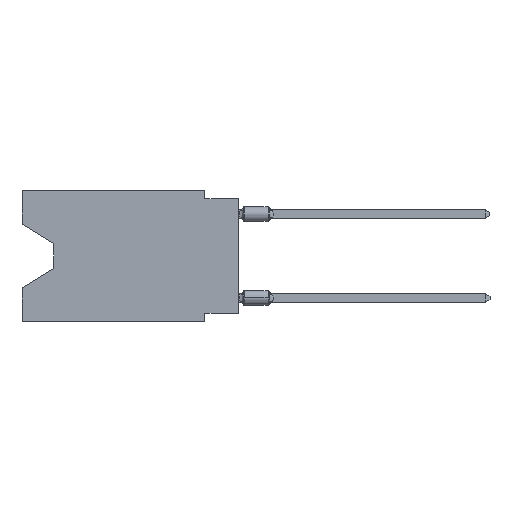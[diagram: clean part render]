
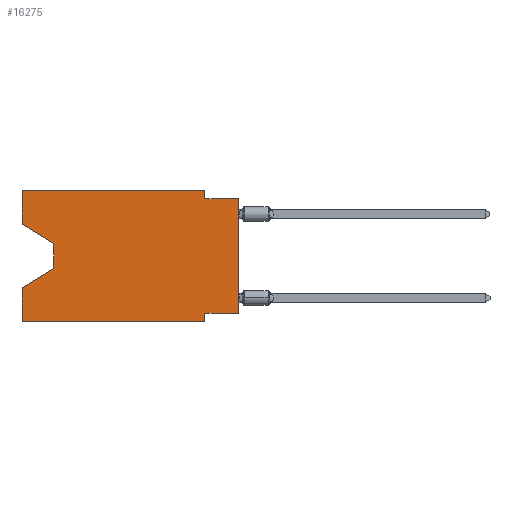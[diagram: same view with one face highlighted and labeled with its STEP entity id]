
A CAD part, left-side view. The second image highlights one B-rep face of the part: STEP entity #16275.
In plain terms, the highlighted planar face has unit normal (-1, 0, 0).
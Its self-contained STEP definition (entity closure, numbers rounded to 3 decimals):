
#249 = PLANE ( 'NONE',  #9242 ) ;
#339 = DIRECTION ( 'NONE',  ( 0., 0., 1. ) ) ;
#496 = CARTESIAN_POINT ( 'NONE',  ( 0., 2.54, -9.906 ) ) ;
#578 = LINE ( 'NONE', #17712, #9018 ) ;
#1679 = CARTESIAN_POINT ( 'NONE',  ( 0., 16.383, 0. ) ) ;
#2886 = EDGE_CURVE ( 'NONE', #3172, #21950, #13737, .T. ) ;
#3172 = VERTEX_POINT ( 'NONE', #18987 ) ;
#3490 = ORIENTED_EDGE ( 'NONE', *, *, #15103, .T. ) ;
#3615 = LINE ( 'NONE', #1679, #9831 ) ;
#3738 = CARTESIAN_POINT ( 'NONE',  ( 0., 0., 0. ) ) ;
#3772 = CARTESIAN_POINT ( 'NONE',  ( 0., 13.97, -4.013 ) ) ;
#3901 = CARTESIAN_POINT ( 'NONE',  ( 0., 16.383, 0. ) ) ;
#4008 = ORIENTED_EDGE ( 'NONE', *, *, #5874, .F. ) ;
#4111 = VECTOR ( 'NONE', #16058, 1000. ) ;
#4529 = CARTESIAN_POINT ( 'NONE',  ( 0., 0., -9.271 ) ) ;
#4678 = DIRECTION ( 'NONE',  ( 0., 0., -1. ) ) ;
#5104 = VECTOR ( 'NONE', #5360, 1000. ) ;
#5166 = CARTESIAN_POINT ( 'NONE',  ( 0., 16.383, 0. ) ) ;
#5337 = VECTOR ( 'NONE', #9088, 1000. ) ;
#5360 = DIRECTION ( 'NONE',  ( 0., -0.855, -0.519 ) ) ;
#5420 = EDGE_CURVE ( 'NONE', #3172, #15425, #14476, .T. ) ;
#5471 = DIRECTION ( 'NONE',  ( 0., 0., -1. ) ) ;
#5735 = DIRECTION ( 'NONE',  ( 1., 0., 0. ) ) ;
#5796 = CARTESIAN_POINT ( 'NONE',  ( 0., 2.54, 0. ) ) ;
#5874 = EDGE_CURVE ( 'NONE', #21510, #11954, #22723, .T. ) ;
#6277 = CARTESIAN_POINT ( 'NONE',  ( 0., 13.97, -4.013 ) ) ;
#6551 = EDGE_CURVE ( 'NONE', #12449, #8440, #20312, .T. ) ;
#7234 = ORIENTED_EDGE ( 'NONE', *, *, #23319, .F. ) ;
#7327 = LINE ( 'NONE', #12842, #19570 ) ;
#7402 = DIRECTION ( 'NONE',  ( 0., 1., 0. ) ) ;
#7459 = VERTEX_POINT ( 'NONE', #9820 ) ;
#7668 = DIRECTION ( 'NONE',  ( 0., 0., 1. ) ) ;
#7743 = ORIENTED_EDGE ( 'NONE', *, *, #16140, .T. ) ;
#7904 = ORIENTED_EDGE ( 'NONE', *, *, #10809, .T. ) ;
#7913 = LINE ( 'NONE', #3738, #8195 ) ;
#8195 = VECTOR ( 'NONE', #7668, 1000. ) ;
#8241 = LINE ( 'NONE', #6277, #9632 ) ;
#8387 = DIRECTION ( 'NONE',  ( 0., 0., -1. ) ) ;
#8440 = VERTEX_POINT ( 'NONE', #18063 ) ;
#8969 = FACE_OUTER_BOUND ( 'NONE', #14209, .T. ) ;
#9018 = VECTOR ( 'NONE', #8387, 1000. ) ;
#9088 = DIRECTION ( 'NONE',  ( 0., 0., 1. ) ) ;
#9242 = AXIS2_PLACEMENT_3D ( 'NONE', #3901, #5735, #16195 ) ;
#9350 = CARTESIAN_POINT ( 'NONE',  ( 0., 16.383, 0. ) ) ;
#9607 = EDGE_CURVE ( 'NONE', #21632, #20937, #3615, .T. ) ;
#9632 = VECTOR ( 'NONE', #4678, 1000. ) ;
#9792 = ORIENTED_EDGE ( 'NONE', *, *, #2886, .T. ) ;
#9820 = CARTESIAN_POINT ( 'NONE',  ( 0., 13.97, -5.893 ) ) ;
#9831 = VECTOR ( 'NONE', #339, 1000. ) ;
#10738 = CARTESIAN_POINT ( 'NONE',  ( 0., 2.54, 0. ) ) ;
#10809 = EDGE_CURVE ( 'NONE', #21510, #15118, #7913, .T. ) ;
#11954 = VERTEX_POINT ( 'NONE', #16613 ) ;
#12120 = EDGE_CURVE ( 'NONE', #11954, #21950, #578, .T. ) ;
#12449 = VERTEX_POINT ( 'NONE', #5796 ) ;
#12842 = CARTESIAN_POINT ( 'NONE',  ( 0., 13.97, -5.893 ) ) ;
#12942 = CARTESIAN_POINT ( 'NONE',  ( 0., 16.383, 0. ) ) ;
#13195 = ORIENTED_EDGE ( 'NONE', *, *, #6551, .F. ) ;
#13737 = LINE ( 'NONE', #19369, #4111 ) ;
#13801 = CARTESIAN_POINT ( 'NONE',  ( 0., 0., -0.635 ) ) ;
#14194 = CARTESIAN_POINT ( 'NONE',  ( 0., 16.383, -2.546 ) ) ;
#14209 = EDGE_LOOP ( 'NONE', ( #14927, #7743, #3490, #22213, #9792, #15461, #4008, #7904, #7234, #13195, #16245, #23745 ) ) ;
#14289 = LINE ( 'NONE', #21651, #19022 ) ;
#14476 = LINE ( 'NONE', #5166, #5337 ) ;
#14860 = LINE ( 'NONE', #9350, #22953 ) ;
#14927 = ORIENTED_EDGE ( 'NONE', *, *, #15098, .T. ) ;
#15098 = EDGE_CURVE ( 'NONE', #21632, #16340, #22157, .T. ) ;
#15103 = EDGE_CURVE ( 'NONE', #7459, #15425, #7327, .T. ) ;
#15106 = CARTESIAN_POINT ( 'NONE',  ( 0., 0., -9.271 ) ) ;
#15118 = VERTEX_POINT ( 'NONE', #13801 ) ;
#15425 = VERTEX_POINT ( 'NONE', #18330 ) ;
#15461 = ORIENTED_EDGE ( 'NONE', *, *, #12120, .F. ) ;
#16058 = DIRECTION ( 'NONE',  ( 0., -1., 0. ) ) ;
#16140 = EDGE_CURVE ( 'NONE', #16340, #7459, #8241, .T. ) ;
#16195 = DIRECTION ( 'NONE',  ( 0., 0., -1. ) ) ;
#16245 = ORIENTED_EDGE ( 'NONE', *, *, #23895, .F. ) ;
#16275 = ADVANCED_FACE ( 'NONE', ( #8969 ), #249, .F. ) ;
#16340 = VERTEX_POINT ( 'NONE', #3772 ) ;
#16613 = CARTESIAN_POINT ( 'NONE',  ( 0., 2.54, -9.271 ) ) ;
#17712 = CARTESIAN_POINT ( 'NONE',  ( 0., 2.54, -9.906 ) ) ;
#17722 = VECTOR ( 'NONE', #7402, 1000. ) ;
#18063 = CARTESIAN_POINT ( 'NONE',  ( 0., 2.54, -0.635 ) ) ;
#18330 = CARTESIAN_POINT ( 'NONE',  ( 0., 16.383, -7.36 ) ) ;
#18482 = CARTESIAN_POINT ( 'NONE',  ( 0., 16.383, -2.546 ) ) ;
#18987 = CARTESIAN_POINT ( 'NONE',  ( 0., 16.383, -9.906 ) ) ;
#19022 = VECTOR ( 'NONE', #20305, 1000. ) ;
#19369 = CARTESIAN_POINT ( 'NONE',  ( 0., 16.383, -9.906 ) ) ;
#19570 = VECTOR ( 'NONE', #22287, 1000. ) ;
#20305 = DIRECTION ( 'NONE',  ( 0., -1., 0. ) ) ;
#20312 = LINE ( 'NONE', #10738, #24004 ) ;
#20762 = DIRECTION ( 'NONE',  ( 0., -1., 0. ) ) ;
#20937 = VERTEX_POINT ( 'NONE', #12942 ) ;
#21510 = VERTEX_POINT ( 'NONE', #4529 ) ;
#21632 = VERTEX_POINT ( 'NONE', #14194 ) ;
#21651 = CARTESIAN_POINT ( 'NONE',  ( 0., 0., -0.635 ) ) ;
#21950 = VERTEX_POINT ( 'NONE', #496 ) ;
#22157 = LINE ( 'NONE', #18482, #5104 ) ;
#22213 = ORIENTED_EDGE ( 'NONE', *, *, #5420, .F. ) ;
#22287 = DIRECTION ( 'NONE',  ( 0., 0.855, -0.519 ) ) ;
#22723 = LINE ( 'NONE', #15106, #17722 ) ;
#22953 = VECTOR ( 'NONE', #20762, 1000. ) ;
#23319 = EDGE_CURVE ( 'NONE', #8440, #15118, #14289, .T. ) ;
#23745 = ORIENTED_EDGE ( 'NONE', *, *, #9607, .F. ) ;
#23895 = EDGE_CURVE ( 'NONE', #20937, #12449, #14860, .T. ) ;
#24004 = VECTOR ( 'NONE', #5471, 1000. ) ;
